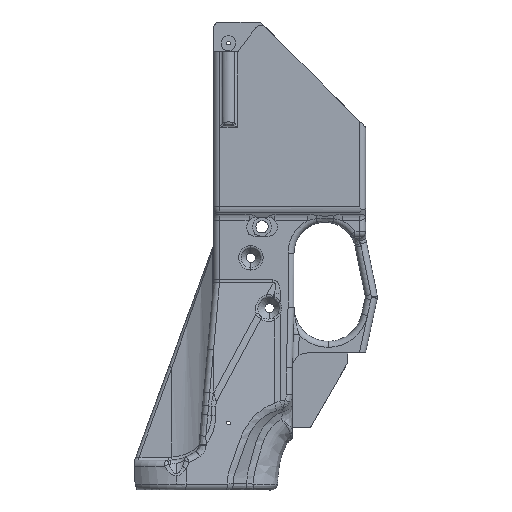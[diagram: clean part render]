
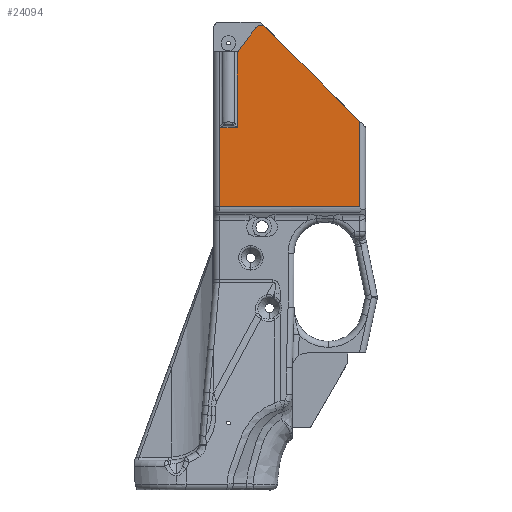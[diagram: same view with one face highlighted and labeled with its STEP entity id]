
A CAD part, left-side view. The second image highlights one B-rep face of the part: STEP entity #24094.
In plain terms, the highlighted planar face has unit normal (-1, 0, 0).
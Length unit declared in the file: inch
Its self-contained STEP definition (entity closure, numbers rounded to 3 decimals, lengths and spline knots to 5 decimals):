
#738 = LINE ( 'NONE', #740, #20979 ) ;
#739 = CARTESIAN_POINT ( 'NONE',  ( 0.2325, -0.98741, 0.95285 ) ) ;
#740 = CARTESIAN_POINT ( 'NONE',  ( 0.2325, -2.5, 0.29672 ) ) ;
#741 = DIRECTION ( 'NONE',  ( 0., -1., 0. ) ) ;
#742 = LINE ( 'NONE', #739, #20980 ) ;
#743 = CARTESIAN_POINT ( 'NONE',  ( 0.2325, -0.53869, 0.19672 ) ) ;
#744 = DIRECTION ( 'NONE',  ( -1., 0., 0. ) ) ;
#745 = DIRECTION ( 'NONE',  ( 0., 0., 1. ) ) ;
#746 = CARTESIAN_POINT ( 'NONE',  ( 0.2325, -2.5, -0.145 ) ) ;
#747 = DIRECTION ( 'NONE',  ( 0., -0.605, 0.796 ) ) ;
#749 = LINE ( 'NONE', #756, #20984 ) ;
#750 = LINE ( 'NONE', #746, #20983 ) ;
#751 = CARTESIAN_POINT ( 'NONE',  ( 0.2325, 0., 0. ) ) ;
#752 = DIRECTION ( 'NONE',  ( -1., 0., 0. ) ) ;
#753 = DIRECTION ( 'NONE',  ( 0., 0., 1. ) ) ;
#755 = DIRECTION ( 'NONE',  ( 0., -1., 0. ) ) ;
#756 = CARTESIAN_POINT ( 'NONE',  ( 0.2325, -0.14325, -1.42 ) ) ;
#757 = DIRECTION ( 'NONE',  ( 0., 0., -1. ) ) ;
#758 = LINE ( 'NONE', #759, #20987 ) ;
#759 = CARTESIAN_POINT ( 'NONE',  ( 0.2325, -2.5, -1.42 ) ) ;
#760 = DIRECTION ( 'NONE',  ( 0., 1., 0. ) ) ;
#761 = LINE ( 'NONE', #762, #20988 ) ;
#762 = CARTESIAN_POINT ( 'NONE',  ( 0.2325, 0.14325, -0.145 ) ) ;
#763 = DIRECTION ( 'NONE',  ( 0., 0., 1. ) ) ;
#764 = LINE ( 'NONE', #765, #20989 ) ;
#765 = CARTESIAN_POINT ( 'NONE',  ( 0.2325, -2.5, -0.145 ) ) ;
#766 = DIRECTION ( 'NONE',  ( 0., -1., 0. ) ) ;
#767 = LINE ( 'NONE', #768, #20990 ) ;
#768 = CARTESIAN_POINT ( 'NONE',  ( 0.2325, 0.15, -2.74584 ) ) ;
#769 = DIRECTION ( 'NONE',  ( 0., 0., -1. ) ) ;
#770 = LINE ( 'NONE', #771, #20991 ) ;
#771 = CARTESIAN_POINT ( 'NONE',  ( 0.2325, -2.5, -2.74584 ) ) ;
#772 = DIRECTION ( 'NONE',  ( 0., -1., 0. ) ) ;
#773 = LINE ( 'NONE', #774, #20992 ) ;
#774 = CARTESIAN_POINT ( 'NONE',  ( 0.2325, -2.2, -1.41421 ) ) ;
#775 = DIRECTION ( 'NONE',  ( 0., 0., 1. ) ) ;
#2662 = CARTESIAN_POINT ( 'NONE',  ( 0.2325, -0.1519, -0.145 ) ) ;
#2676 = CARTESIAN_POINT ( 'NONE',  ( 0.2325, -0.53869, 0.29672 ) ) ;
#2677 = CARTESIAN_POINT ( 'NONE',  ( 0.2325, -0.16723, -0.12702 ) ) ;
#2680 = CARTESIAN_POINT ( 'NONE',  ( 0.2325, -0.14325, -0.145 ) ) ;
#2681 = CARTESIAN_POINT ( 'NONE',  ( 0.2325, -0.45905, 0.2572 ) ) ;
#2684 = CARTESIAN_POINT ( 'NONE',  ( 0.2325, 0.15, -0.145 ) ) ;
#2685 = CARTESIAN_POINT ( 'NONE',  ( 0.2325, -0.14325, -1.42 ) ) ;
#2686 = CARTESIAN_POINT ( 'NONE',  ( 0.2325, 0.14325, -1.42 ) ) ;
#2687 = CARTESIAN_POINT ( 'NONE',  ( 0.2325, 0.14325, -0.145 ) ) ;
#2689 = CARTESIAN_POINT ( 'NONE',  ( 0.2325, 0.15, -2.74584 ) ) ;
#2690 = CARTESIAN_POINT ( 'NONE',  ( 0.2325, -2.2, -2.74584 ) ) ;
#3941 = CARTESIAN_POINT ( 'NONE',  ( 0.2325, -2.5, -0.19599 ) ) ;
#3949 = FACE_OUTER_BOUND ( 'NONE', #26118, .T. ) ;
#3950 = PLANE ( 'NONE',  #39618 ) ;
#3952 = DIRECTION ( 'NONE',  ( -1., 0., 0. ) ) ;
#3953 = DIRECTION ( 'NONE',  ( 0., 0., 1. ) ) ;
#7360 = EDGE_CURVE ( 'NONE', #11294, #10918, #738, .T. ) ;
#7361 = EDGE_CURVE ( 'NONE', #11294, #11299, #20975, .T. ) ;
#7362 = EDGE_CURVE ( 'NONE', #11295, #11299, #742, .T. ) ;
#7363 = EDGE_CURVE ( 'NONE', #11280, #11295, #20981, .T. ) ;
#7364 = EDGE_CURVE ( 'NONE', #11298, #11280, #750, .T. ) ;
#7365 = EDGE_CURVE ( 'NONE', #11298, #11303, #749, .T. ) ;
#7366 = EDGE_CURVE ( 'NONE', #11303, #11304, #758, .T. ) ;
#7367 = EDGE_CURVE ( 'NONE', #11304, #11305, #761, .T. ) ;
#7368 = EDGE_CURVE ( 'NONE', #11302, #11305, #764, .T. ) ;
#7369 = EDGE_CURVE ( 'NONE', #11302, #11307, #767, .T. ) ;
#7370 = EDGE_CURVE ( 'NONE', #11307, #11308, #770, .T. ) ;
#7371 = EDGE_CURVE ( 'NONE', #11308, #10919, #773, .T. ) ;
#10918 = VERTEX_POINT ( 'NONE', #36936 ) ;
#10919 = VERTEX_POINT ( 'NONE', #36938 ) ;
#11280 = VERTEX_POINT ( 'NONE', #2662 ) ;
#11294 = VERTEX_POINT ( 'NONE', #2676 ) ;
#11295 = VERTEX_POINT ( 'NONE', #2677 ) ;
#11298 = VERTEX_POINT ( 'NONE', #2680 ) ;
#11299 = VERTEX_POINT ( 'NONE', #2681 ) ;
#11302 = VERTEX_POINT ( 'NONE', #2684 ) ;
#11303 = VERTEX_POINT ( 'NONE', #2685 ) ;
#11304 = VERTEX_POINT ( 'NONE', #2686 ) ;
#11305 = VERTEX_POINT ( 'NONE', #2687 ) ;
#11307 = VERTEX_POINT ( 'NONE', #2689 ) ;
#11308 = VERTEX_POINT ( 'NONE', #2690 ) ;
#16342 = LINE ( 'NONE', #16343, #38797 ) ;
#16343 = CARTESIAN_POINT ( 'NONE',  ( 0.2325, -2.3, -1.41421 ) ) ;
#16344 = DIRECTION ( 'NONE',  ( 0., 0.707, 0.707 ) ) ;
#20975 = CIRCLE ( 'NONE', #20982, 0.1 ) ;
#20979 = VECTOR ( 'NONE', #741, 39.37008 ) ;
#20980 = VECTOR ( 'NONE', #747, 39.37008 ) ;
#20981 = CIRCLE ( 'NONE', #20985, 0.21 ) ;
#20982 = AXIS2_PLACEMENT_3D ( 'NONE', #743, #744, #745 ) ;
#20983 = VECTOR ( 'NONE', #755, 39.37008 ) ;
#20984 = VECTOR ( 'NONE', #757, 39.37008 ) ;
#20985 = AXIS2_PLACEMENT_3D ( 'NONE', #751, #752, #753 ) ;
#20987 = VECTOR ( 'NONE', #760, 39.37008 ) ;
#20988 = VECTOR ( 'NONE', #763, 39.37008 ) ;
#20989 = VECTOR ( 'NONE', #766, 39.37008 ) ;
#20990 = VECTOR ( 'NONE', #769, 39.37008 ) ;
#20991 = VECTOR ( 'NONE', #772, 39.37008 ) ;
#20992 = VECTOR ( 'NONE', #775, 39.37008 ) ;
#22147 = EDGE_CURVE ( 'NONE', #10919, #10918, #16342, .T. ) ;
#24094 = ADVANCED_FACE ( 'NONE', ( #3949 ), #3950, .T. ) ;
#26118 = EDGE_LOOP ( 'NONE', ( #30846, #30798, #31379, #30917, #31266, #31330, #31161, #31088, #30811, #30766, #30866, #31333, #30858 ) ) ;
#30766 = ORIENTED_EDGE ( 'NONE', *, *, #7369, .T. ) ;
#30798 = ORIENTED_EDGE ( 'NONE', *, *, #7361, .T. ) ;
#30811 = ORIENTED_EDGE ( 'NONE', *, *, #7368, .F. ) ;
#30846 = ORIENTED_EDGE ( 'NONE', *, *, #7360, .F. ) ;
#30858 = ORIENTED_EDGE ( 'NONE', *, *, #22147, .T. ) ;
#30866 = ORIENTED_EDGE ( 'NONE', *, *, #7370, .T. ) ;
#30917 = ORIENTED_EDGE ( 'NONE', *, *, #7363, .F. ) ;
#31088 = ORIENTED_EDGE ( 'NONE', *, *, #7367, .T. ) ;
#31161 = ORIENTED_EDGE ( 'NONE', *, *, #7366, .T. ) ;
#31266 = ORIENTED_EDGE ( 'NONE', *, *, #7364, .F. ) ;
#31330 = ORIENTED_EDGE ( 'NONE', *, *, #7365, .T. ) ;
#31333 = ORIENTED_EDGE ( 'NONE', *, *, #7371, .T. ) ;
#31379 = ORIENTED_EDGE ( 'NONE', *, *, #7362, .F. ) ;
#36936 = CARTESIAN_POINT ( 'NONE',  ( 0.2325, -0.58907, 0.29672 ) ) ;
#36938 = CARTESIAN_POINT ( 'NONE',  ( 0.2325, -2.2, -1.31421 ) ) ;
#38797 = VECTOR ( 'NONE', #16344, 39.37008 ) ;
#39618 = AXIS2_PLACEMENT_3D ( 'NONE', #3941, #3952, #3953 ) ;
